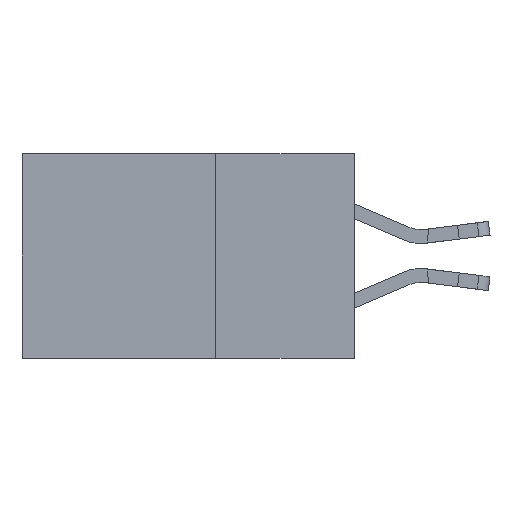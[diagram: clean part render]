
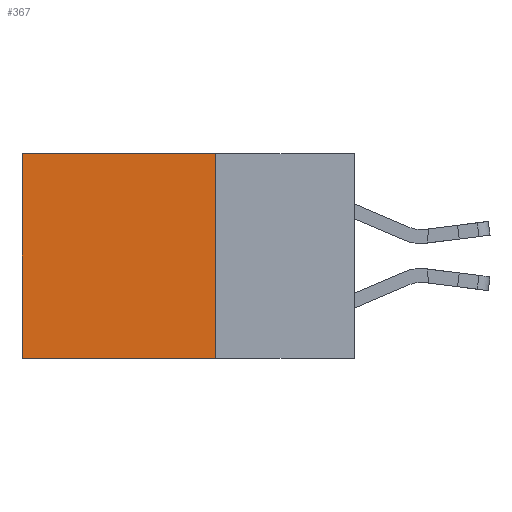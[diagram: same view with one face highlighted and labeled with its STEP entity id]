
A CAD part, left-side view. The second image highlights one B-rep face of the part: STEP entity #367.
In plain terms, the highlighted planar face has unit normal (-1, 0, 0).
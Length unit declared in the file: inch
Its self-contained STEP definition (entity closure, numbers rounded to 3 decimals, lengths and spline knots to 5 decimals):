
#68 = DIRECTION ( 'NONE',  ( 0., 0., -1. ) ) ;
#104 = EDGE_CURVE ( 'NONE', #4698, #5798, #10972, .T. ) ;
#367 = ADVANCED_FACE ( 'NONE', ( #5620 ), #7167, .F. ) ;
#1516 = DIRECTION ( 'NONE',  ( 0., 1., 0. ) ) ;
#1560 = VECTOR ( 'NONE', #1516, 39.37008 ) ;
#1755 = CARTESIAN_POINT ( 'NONE',  ( 0.298, 0.25, 0. ) ) ;
#2411 = DIRECTION ( 'NONE',  ( 1., 0., 0. ) ) ;
#2460 = VECTOR ( 'NONE', #7419, 39.37008 ) ;
#2610 = EDGE_CURVE ( 'NONE', #7194, #5877, #5711, .T. ) ;
#2864 = CARTESIAN_POINT ( 'NONE',  ( 0.298, 0.25, 0. ) ) ;
#3106 = AXIS2_PLACEMENT_3D ( 'NONE', #10979, #2411, #3264 ) ;
#3264 = DIRECTION ( 'NONE',  ( 0., 0., -1. ) ) ;
#3475 = CARTESIAN_POINT ( 'NONE',  ( 0.298, 0.6, 0. ) ) ;
#3838 = ORIENTED_EDGE ( 'NONE', *, *, #9716, .T. ) ;
#3874 = DIRECTION ( 'NONE',  ( 0., 1., 0. ) ) ;
#4062 = LINE ( 'NONE', #7686, #5981 ) ;
#4698 = VERTEX_POINT ( 'NONE', #3475 ) ;
#4817 = CARTESIAN_POINT ( 'NONE',  ( 0.298, 0.6, 0. ) ) ;
#5547 = LINE ( 'NONE', #11079, #1560 ) ;
#5620 = FACE_OUTER_BOUND ( 'NONE', #8795, .T. ) ;
#5629 = VECTOR ( 'NONE', #68, 39.37008 ) ;
#5711 = LINE ( 'NONE', #1755, #2460 ) ;
#5798 = VERTEX_POINT ( 'NONE', #7769 ) ;
#5877 = VERTEX_POINT ( 'NONE', #9559 ) ;
#5981 = VECTOR ( 'NONE', #3874, 39.37008 ) ;
#7167 = PLANE ( 'NONE',  #3106 ) ;
#7194 = VERTEX_POINT ( 'NONE', #2864 ) ;
#7419 = DIRECTION ( 'NONE',  ( 0., 0., -1. ) ) ;
#7686 = CARTESIAN_POINT ( 'NONE',  ( 0.298, 0.25, -0.37 ) ) ;
#7769 = CARTESIAN_POINT ( 'NONE',  ( 0.298, 0.6, -0.37 ) ) ;
#8248 = ORIENTED_EDGE ( 'NONE', *, *, #104, .T. ) ;
#8795 = EDGE_LOOP ( 'NONE', ( #8248, #11215, #11902, #3838 ) ) ;
#8875 = EDGE_CURVE ( 'NONE', #5877, #5798, #4062, .T. ) ;
#9559 = CARTESIAN_POINT ( 'NONE',  ( 0.298, 0.25, -0.37 ) ) ;
#9716 = EDGE_CURVE ( 'NONE', #7194, #4698, #5547, .T. ) ;
#10972 = LINE ( 'NONE', #4817, #5629 ) ;
#10979 = CARTESIAN_POINT ( 'NONE',  ( 0.298, 0.25, 0. ) ) ;
#11079 = CARTESIAN_POINT ( 'NONE',  ( 0.298, 0.25, 0. ) ) ;
#11215 = ORIENTED_EDGE ( 'NONE', *, *, #8875, .F. ) ;
#11902 = ORIENTED_EDGE ( 'NONE', *, *, #2610, .F. ) ;
